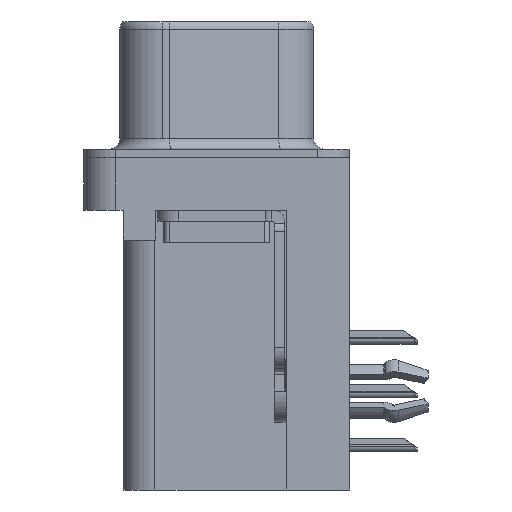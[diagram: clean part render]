
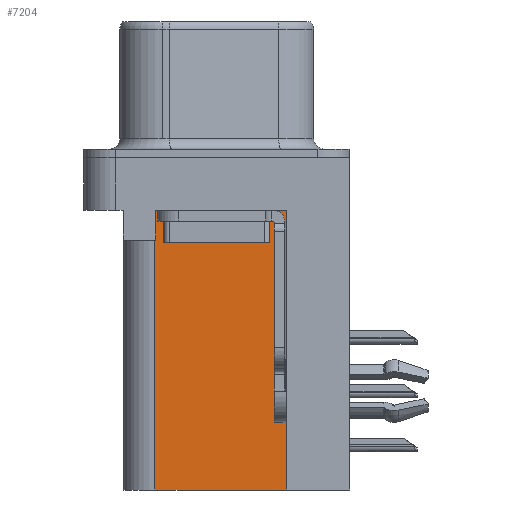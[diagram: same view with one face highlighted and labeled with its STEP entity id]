
A CAD part, left-side view. The second image highlights one B-rep face of the part: STEP entity #7204.
In plain terms, the highlighted planar face has unit normal (-1, 0, 0).
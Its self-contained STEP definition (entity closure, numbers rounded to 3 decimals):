
#132 = AXIS2_PLACEMENT_3D ( 'NONE', #25797, #6482, #23507 ) ;
#190 = CARTESIAN_POINT ( 'NONE',  ( 3.7, 2.925, -15.7 ) ) ;
#391 = EDGE_LOOP ( 'NONE', ( #18439, #19795, #20890, #28832, #1512, #7829 ) ) ;
#416 = DIRECTION ( 'NONE',  ( 0., 0., 1. ) ) ;
#635 = LINE ( 'NONE', #11728, #12935 ) ;
#1512 = ORIENTED_EDGE ( 'NONE', *, *, #9450, .F. ) ;
#1609 = EDGE_CURVE ( 'NONE', #30345, #9645, #21354, .T. ) ;
#2155 = DIRECTION ( 'NONE',  ( 0., 1., 0. ) ) ;
#4386 = DIRECTION ( 'NONE',  ( 0., 0., -1. ) ) ;
#4509 = DIRECTION ( 'NONE',  ( 0., 1., 0. ) ) ;
#4852 = LINE ( 'NONE', #17432, #10569 ) ;
#5309 = DIRECTION ( 'NONE',  ( 0., 0., 1. ) ) ;
#6482 = DIRECTION ( 'NONE',  ( 1., 0., 0. ) ) ;
#6577 = CARTESIAN_POINT ( 'NONE',  ( 3.7, -3.295, -15.7 ) ) ;
#6738 = CARTESIAN_POINT ( 'NONE',  ( 3.7, 2.895, -3.9 ) ) ;
#7204 = ADVANCED_FACE ( 'NONE', ( #25015 ), #21037, .F. ) ;
#7266 = VECTOR ( 'NONE', #4386, 1000. ) ;
#7829 = ORIENTED_EDGE ( 'NONE', *, *, #29549, .T. ) ;
#8239 = EDGE_CURVE ( 'NONE', #9733, #11009, #12818, .T. ) ;
#8450 = CARTESIAN_POINT ( 'NONE',  ( 3.7, 2.895, -3.9 ) ) ;
#9450 = EDGE_CURVE ( 'NONE', #21877, #30345, #635, .T. ) ;
#9593 = VECTOR ( 'NONE', #2155, 1000. ) ;
#9645 = VERTEX_POINT ( 'NONE', #15026 ) ;
#9733 = VERTEX_POINT ( 'NONE', #29959 ) ;
#10569 = VECTOR ( 'NONE', #5309, 1000. ) ;
#11009 = VERTEX_POINT ( 'NONE', #23918 ) ;
#11118 = CARTESIAN_POINT ( 'NONE',  ( 3.7, 2.925, -15.7 ) ) ;
#11728 = CARTESIAN_POINT ( 'NONE',  ( 3.7, -3.295, -15.7 ) ) ;
#12058 = VECTOR ( 'NONE', #17106, 1000. ) ;
#12818 = LINE ( 'NONE', #31644, #12058 ) ;
#12935 = VECTOR ( 'NONE', #4509, 1000. ) ;
#14141 = VECTOR ( 'NONE', #416, 1000. ) ;
#15026 = CARTESIAN_POINT ( 'NONE',  ( 3.7, 2.925, -3.9 ) ) ;
#16045 = LINE ( 'NONE', #31337, #9593 ) ;
#17106 = DIRECTION ( 'NONE',  ( 0., 1., 0. ) ) ;
#17432 = CARTESIAN_POINT ( 'NONE',  ( 3.7, -3.295, -15.7 ) ) ;
#18439 = ORIENTED_EDGE ( 'NONE', *, *, #8239, .T. ) ;
#19795 = ORIENTED_EDGE ( 'NONE', *, *, #27349, .T. ) ;
#20890 = ORIENTED_EDGE ( 'NONE', *, *, #26748, .T. ) ;
#21037 = PLANE ( 'NONE',  #132 ) ;
#21354 = LINE ( 'NONE', #190, #14141 ) ;
#21877 = VERTEX_POINT ( 'NONE', #6577 ) ;
#23507 = DIRECTION ( 'NONE',  ( 0., 0., -1. ) ) ;
#23918 = CARTESIAN_POINT ( 'NONE',  ( 3.7, 2.895, -2.5 ) ) ;
#24165 = VERTEX_POINT ( 'NONE', #8450 ) ;
#25015 = FACE_OUTER_BOUND ( 'NONE', #391, .T. ) ;
#25797 = CARTESIAN_POINT ( 'NONE',  ( 3.7, -3.295, -15.7 ) ) ;
#26628 = LINE ( 'NONE', #6738, #7266 ) ;
#26748 = EDGE_CURVE ( 'NONE', #24165, #9645, #16045, .T. ) ;
#27349 = EDGE_CURVE ( 'NONE', #11009, #24165, #26628, .T. ) ;
#28832 = ORIENTED_EDGE ( 'NONE', *, *, #1609, .F. ) ;
#29549 = EDGE_CURVE ( 'NONE', #21877, #9733, #4852, .T. ) ;
#29959 = CARTESIAN_POINT ( 'NONE',  ( 3.7, -3.295, -2.5 ) ) ;
#30345 = VERTEX_POINT ( 'NONE', #11118 ) ;
#31337 = CARTESIAN_POINT ( 'NONE',  ( 3.7, 0., -3.9 ) ) ;
#31644 = CARTESIAN_POINT ( 'NONE',  ( 3.7, -3.295, -2.5 ) ) ;
